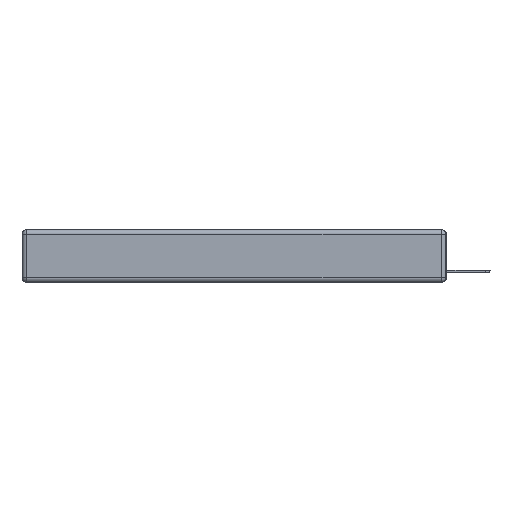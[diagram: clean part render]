
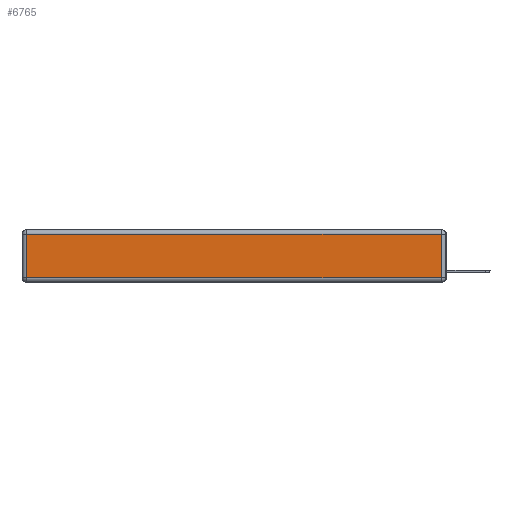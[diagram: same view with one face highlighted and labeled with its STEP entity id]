
A CAD part, left-side view. The second image highlights one B-rep face of the part: STEP entity #6765.
In plain terms, the highlighted planar face has unit normal (-1, 0, 0).
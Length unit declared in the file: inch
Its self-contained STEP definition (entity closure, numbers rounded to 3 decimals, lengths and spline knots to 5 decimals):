
#194 = DIRECTION ( 'NONE',  ( 0., 1., 0. ) ) ;
#255 = ORIENTED_EDGE ( 'NONE', *, *, #15330, .T. ) ;
#845 = VERTEX_POINT ( 'NONE', #5864 ) ;
#1637 = VECTOR ( 'NONE', #4895, 39.37008 ) ;
#1731 = ORIENTED_EDGE ( 'NONE', *, *, #19466, .T. ) ;
#1800 = DIRECTION ( 'NONE',  ( -1., 0., 0. ) ) ;
#2060 = EDGE_CURVE ( 'NONE', #16717, #20198, #2850, .T. ) ;
#2850 = LINE ( 'NONE', #20371, #18907 ) ;
#3954 = VECTOR ( 'NONE', #9445, 39.37008 ) ;
#4357 = CARTESIAN_POINT ( 'NONE',  ( 0., 2.72, -0.03 ) ) ;
#4895 = DIRECTION ( 'NONE',  ( 0., 0., -1. ) ) ;
#5864 = CARTESIAN_POINT ( 'NONE',  ( 0., 0.03, -0.313 ) ) ;
#6025 = VERTEX_POINT ( 'NONE', #8376 ) ;
#6315 = LINE ( 'NONE', #19551, #3954 ) ;
#6765 = ADVANCED_FACE ( 'NONE', ( #19962 ), #13802, .T. ) ;
#8376 = CARTESIAN_POINT ( 'NONE',  ( 0., 2.72, -0.313 ) ) ;
#8546 = AXIS2_PLACEMENT_3D ( 'NONE', #15354, #1800, #17238 ) ;
#9261 = DIRECTION ( 'NONE',  ( 0., 0., 1. ) ) ;
#9445 = DIRECTION ( 'NONE',  ( 0., -1., 0. ) ) ;
#9572 = ORIENTED_EDGE ( 'NONE', *, *, #11063, .T. ) ;
#9889 = CARTESIAN_POINT ( 'NONE',  ( 0., 0.03, -0.03 ) ) ;
#11063 = EDGE_CURVE ( 'NONE', #6025, #845, #6315, .T. ) ;
#12734 = LINE ( 'NONE', #13769, #19851 ) ;
#13769 = CARTESIAN_POINT ( 'NONE',  ( 0., 0.03, -0.343 ) ) ;
#13802 = PLANE ( 'NONE',  #8546 ) ;
#14290 = LINE ( 'NONE', #21736, #1637 ) ;
#15330 = EDGE_CURVE ( 'NONE', #20198, #6025, #14290, .T. ) ;
#15354 = CARTESIAN_POINT ( 'NONE',  ( 0., 0., -0.343 ) ) ;
#15500 = ORIENTED_EDGE ( 'NONE', *, *, #2060, .T. ) ;
#16717 = VERTEX_POINT ( 'NONE', #9889 ) ;
#17238 = DIRECTION ( 'NONE',  ( 0., 0., 1. ) ) ;
#18907 = VECTOR ( 'NONE', #194, 39.37008 ) ;
#19300 = EDGE_LOOP ( 'NONE', ( #9572, #1731, #15500, #255 ) ) ;
#19466 = EDGE_CURVE ( 'NONE', #845, #16717, #12734, .T. ) ;
#19551 = CARTESIAN_POINT ( 'NONE',  ( 0., 0., -0.313 ) ) ;
#19851 = VECTOR ( 'NONE', #9261, 39.37008 ) ;
#19962 = FACE_OUTER_BOUND ( 'NONE', #19300, .T. ) ;
#20198 = VERTEX_POINT ( 'NONE', #4357 ) ;
#20371 = CARTESIAN_POINT ( 'NONE',  ( 0., 2.75, -0.03 ) ) ;
#21736 = CARTESIAN_POINT ( 'NONE',  ( 0., 2.72, -0.343 ) ) ;
